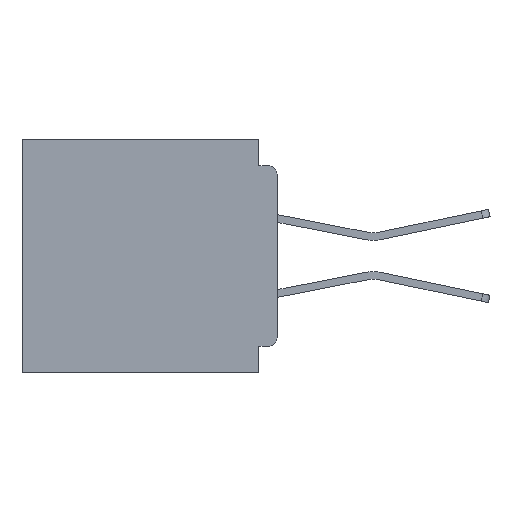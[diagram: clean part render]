
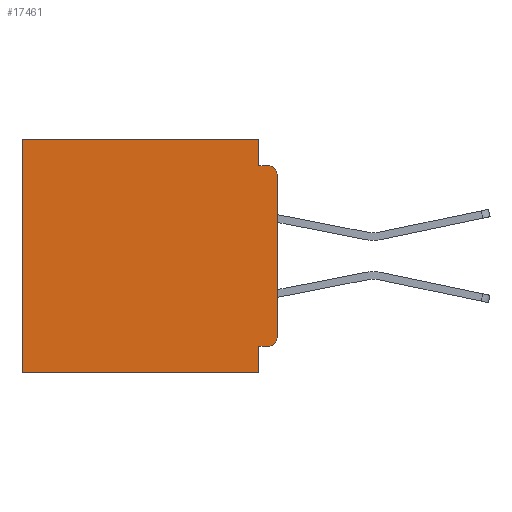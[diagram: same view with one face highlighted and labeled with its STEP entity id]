
A CAD part, left-side view. The second image highlights one B-rep face of the part: STEP entity #17461.
In plain terms, the highlighted planar face has unit normal (-1, 0, 0).
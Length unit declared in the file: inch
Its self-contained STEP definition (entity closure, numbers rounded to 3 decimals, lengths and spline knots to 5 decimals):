
#966 = CARTESIAN_POINT ( 'NONE',  ( 0.3, 0.031, -0.4 ) ) ;
#1530 = DIRECTION ( 'NONE',  ( 0., 0., -1. ) ) ;
#2057 = ORIENTED_EDGE ( 'NONE', *, *, #16484, .F. ) ;
#4016 = LINE ( 'NONE', #966, #53084 ) ;
#4907 = ORIENTED_EDGE ( 'NONE', *, *, #50203, .F. ) ;
#6758 = DIRECTION ( 'NONE',  ( 0., 1., 0. ) ) ;
#7907 = CARTESIAN_POINT ( 'NONE',  ( 0.3, 0.031, 0. ) ) ;
#9210 = CARTESIAN_POINT ( 'NONE',  ( 0.3, 0., -0.045 ) ) ;
#9411 = DIRECTION ( 'NONE',  ( 0., -1., 0. ) ) ;
#9453 = VERTEX_POINT ( 'NONE', #7907 ) ;
#11137 = LINE ( 'NONE', #30056, #49076 ) ;
#11233 = DIRECTION ( 'NONE',  ( 0., 1., 0. ) ) ;
#11464 = EDGE_LOOP ( 'NONE', ( #25174, #58838, #33282, #4907, #33849, #16418, #41959, #2057, #12759, #55994 ) ) ;
#11566 = VERTEX_POINT ( 'NONE', #29153 ) ;
#12651 = EDGE_CURVE ( 'NONE', #38731, #28090, #40226, .T. ) ;
#12759 = ORIENTED_EDGE ( 'NONE', *, *, #25090, .F. ) ;
#13824 = CIRCLE ( 'NONE', #52666, 0.015 ) ;
#13994 = CARTESIAN_POINT ( 'NONE',  ( 0.3, 0.015, -0.06 ) ) ;
#16418 = ORIENTED_EDGE ( 'NONE', *, *, #42094, .T. ) ;
#16484 = EDGE_CURVE ( 'NONE', #11566, #31250, #4016, .T. ) ;
#17461 = ADVANCED_FACE ( 'NONE', ( #47030 ), #17662, .F. ) ;
#17662 = PLANE ( 'NONE',  #32104 ) ;
#17780 = CARTESIAN_POINT ( 'NONE',  ( 0.3, 0.437, 0. ) ) ;
#18154 = DIRECTION ( 'NONE',  ( -1., 0., 0. ) ) ;
#18172 = VERTEX_POINT ( 'NONE', #17780 ) ;
#18430 = VERTEX_POINT ( 'NONE', #29270 ) ;
#18786 = DIRECTION ( 'NONE',  ( 0., 0., -1. ) ) ;
#18858 = VECTOR ( 'NONE', #6758, 39.37008 ) ;
#19044 = EDGE_CURVE ( 'NONE', #39393, #18430, #50548, .T. ) ;
#20545 = LINE ( 'NONE', #43308, #56926 ) ;
#25090 = EDGE_CURVE ( 'NONE', #48896, #11566, #57023, .T. ) ;
#25174 = ORIENTED_EDGE ( 'NONE', *, *, #12651, .F. ) ;
#25299 = VECTOR ( 'NONE', #9411, 39.37008 ) ;
#25373 = VECTOR ( 'NONE', #11233, 39.37008 ) ;
#25437 = CARTESIAN_POINT ( 'NONE',  ( 0.3, 0.031, -0.4 ) ) ;
#25544 = CARTESIAN_POINT ( 'NONE',  ( 0.3, 0.015, -0.355 ) ) ;
#26487 = CIRCLE ( 'NONE', #38128, 0.015 ) ;
#27344 = DIRECTION ( 'NONE',  ( 0., 0., -1. ) ) ;
#27629 = VECTOR ( 'NONE', #27344, 39.37008 ) ;
#28090 = VERTEX_POINT ( 'NONE', #57693 ) ;
#29153 = CARTESIAN_POINT ( 'NONE',  ( 0.3, 0.031, -0.355 ) ) ;
#29270 = CARTESIAN_POINT ( 'NONE',  ( 0.3, 0.015, -0.045 ) ) ;
#29495 = DIRECTION ( 'NONE',  ( 0., 0., -1. ) ) ;
#30055 = LINE ( 'NONE', #35286, #18858 ) ;
#30056 = CARTESIAN_POINT ( 'NONE',  ( 0.3, 0.031, 0. ) ) ;
#30336 = VECTOR ( 'NONE', #49080, 39.37008 ) ;
#31250 = VERTEX_POINT ( 'NONE', #25437 ) ;
#32084 = DIRECTION ( 'NONE',  ( 0., 0., -1. ) ) ;
#32104 = AXIS2_PLACEMENT_3D ( 'NONE', #41413, #60415, #32084 ) ;
#32914 = CARTESIAN_POINT ( 'NONE',  ( 0.3, 0., -0.06 ) ) ;
#33282 = ORIENTED_EDGE ( 'NONE', *, *, #19044, .F. ) ;
#33849 = ORIENTED_EDGE ( 'NONE', *, *, #52711, .T. ) ;
#34765 = CARTESIAN_POINT ( 'NONE',  ( 0.3, 0., 0. ) ) ;
#35286 = CARTESIAN_POINT ( 'NONE',  ( 0.3, 0., -0.4 ) ) ;
#38128 = AXIS2_PLACEMENT_3D ( 'NONE', #46650, #18154, #51432 ) ;
#38731 = VERTEX_POINT ( 'NONE', #32914 ) ;
#39393 = VERTEX_POINT ( 'NONE', #43199 ) ;
#39477 = LINE ( 'NONE', #34765, #25373 ) ;
#40226 = LINE ( 'NONE', #41432, #27629 ) ;
#41413 = CARTESIAN_POINT ( 'NONE',  ( 0.3, 0., -0.4 ) ) ;
#41432 = CARTESIAN_POINT ( 'NONE',  ( 0.3, 0., -0.4 ) ) ;
#41938 = EDGE_CURVE ( 'NONE', #38731, #18430, #13824, .T. ) ;
#41959 = ORIENTED_EDGE ( 'NONE', *, *, #43462, .F. ) ;
#42094 = EDGE_CURVE ( 'NONE', #18172, #43595, #20545, .T. ) ;
#43199 = CARTESIAN_POINT ( 'NONE',  ( 0.3, 0.031, -0.045 ) ) ;
#43308 = CARTESIAN_POINT ( 'NONE',  ( 0.3, 0.437, -0.4 ) ) ;
#43462 = EDGE_CURVE ( 'NONE', #31250, #43595, #30055, .T. ) ;
#43595 = VERTEX_POINT ( 'NONE', #50418 ) ;
#46650 = CARTESIAN_POINT ( 'NONE',  ( 0.3, 0.015, -0.34 ) ) ;
#47030 = FACE_OUTER_BOUND ( 'NONE', #11464, .T. ) ;
#47255 = DIRECTION ( 'NONE',  ( -1., 0., 0. ) ) ;
#48896 = VERTEX_POINT ( 'NONE', #25544 ) ;
#49076 = VECTOR ( 'NONE', #1530, 39.37008 ) ;
#49080 = DIRECTION ( 'NONE',  ( 0., 1., 0. ) ) ;
#50203 = EDGE_CURVE ( 'NONE', #9453, #39393, #11137, .T. ) ;
#50418 = CARTESIAN_POINT ( 'NONE',  ( 0.3, 0.437, -0.4 ) ) ;
#50548 = LINE ( 'NONE', #9210, #25299 ) ;
#51432 = DIRECTION ( 'NONE',  ( 0., 0., -1. ) ) ;
#52666 = AXIS2_PLACEMENT_3D ( 'NONE', #13994, #47255, #18786 ) ;
#52711 = EDGE_CURVE ( 'NONE', #9453, #18172, #39477, .T. ) ;
#52829 = DIRECTION ( 'NONE',  ( 0., 0., -1. ) ) ;
#53084 = VECTOR ( 'NONE', #29495, 39.37008 ) ;
#55746 = EDGE_CURVE ( 'NONE', #48896, #28090, #26487, .T. ) ;
#55994 = ORIENTED_EDGE ( 'NONE', *, *, #55746, .T. ) ;
#56926 = VECTOR ( 'NONE', #52829, 39.37008 ) ;
#57023 = LINE ( 'NONE', #58562, #30336 ) ;
#57693 = CARTESIAN_POINT ( 'NONE',  ( 0.3, 0., -0.34 ) ) ;
#58562 = CARTESIAN_POINT ( 'NONE',  ( 0.3, 0., -0.355 ) ) ;
#58838 = ORIENTED_EDGE ( 'NONE', *, *, #41938, .T. ) ;
#60415 = DIRECTION ( 'NONE',  ( 1., 0., 0. ) ) ;
